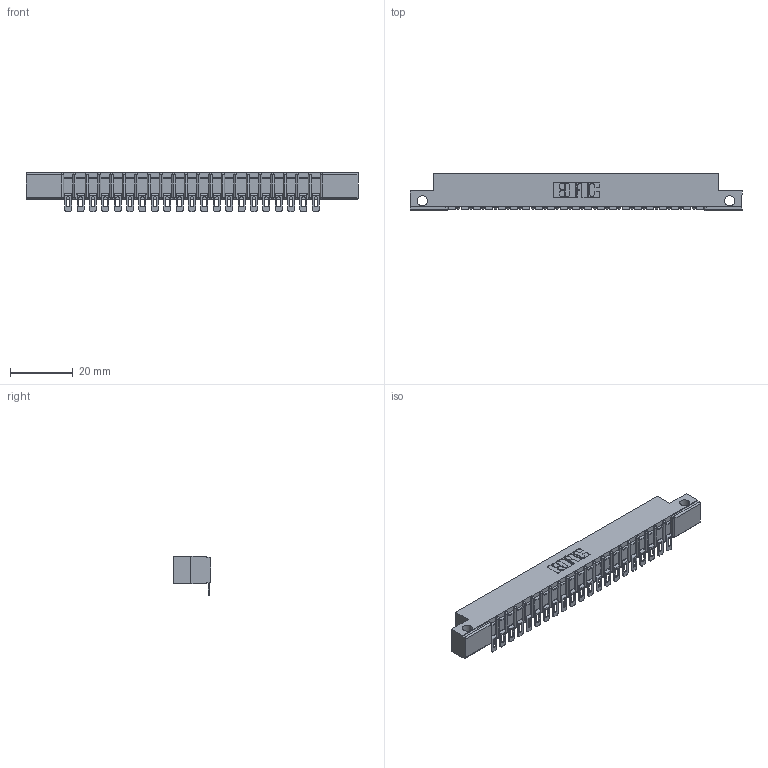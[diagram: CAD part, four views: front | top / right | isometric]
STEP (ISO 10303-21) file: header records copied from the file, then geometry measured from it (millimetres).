
FILE_DESCRIPTION (( 'STEP AP203' ), '1' );
FILE_NAME ('357-021-554-112.STEP', '2019-09-16T22:56:08', ( '' ), ( '' ), 'SwSTEP 2.0', 'SolidWorks 2016', '' );
FILE_SCHEMA (( 'CONFIG_CONTROL_DESIGN' ));
Length unit declared in the file: inch
Products named in the file (3): 357-021-554-112; 307-290-002_554; 307 Part_.128 Dia Side Mounting Holes
Assembly tree (22 placements, depth 2):
  357-021-554-112
    307 Part_.128 Dia Side Mounting Holes
    307-290-002_554  x21
Bounding box: 106.22 x 12.01 x 12.52 mm (x, y, z)
Volume: 6943.8 mm3; surface area: 12522.8 mm2
Topology: 22 solids, 22 shells, 1841 faces, 5636 edges, 3696 vertices
Faces by surface type: plane 1036, cylinder 761, sphere 44
Entity records: 21559 total; most frequent: CARTESIAN_POINT 3634, ORIENTED_EDGE 3624, DIRECTION 3546, EDGE_CURVE 1812, VECTOR 1370, LINE 1370, VERTEX_POINT 1176, AXIS2_PLACEMENT_3D 1088
